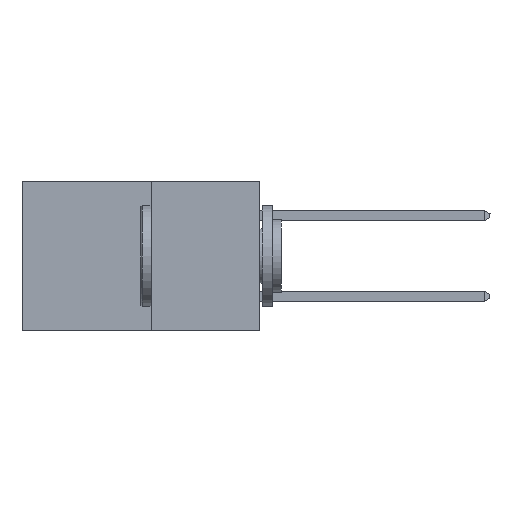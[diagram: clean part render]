
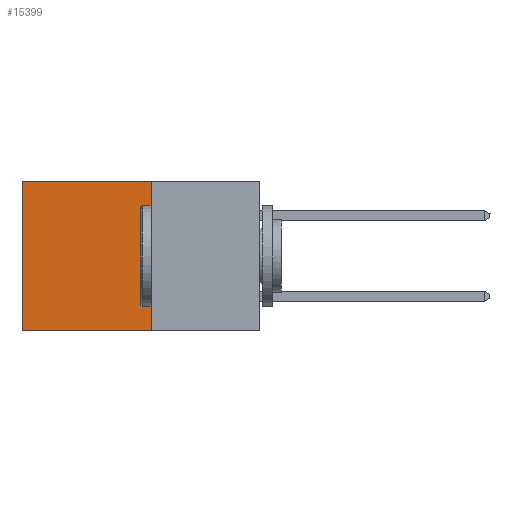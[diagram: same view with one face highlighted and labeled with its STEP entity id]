
A CAD part, left-side view. The second image highlights one B-rep face of the part: STEP entity #15399.
In plain terms, the highlighted planar face has unit normal (-1, 0, 0).
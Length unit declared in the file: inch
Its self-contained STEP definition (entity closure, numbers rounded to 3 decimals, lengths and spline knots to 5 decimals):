
#458 = DIRECTION ( 'NONE',  ( 0., 0., -1. ) ) ;
#594 = VERTEX_POINT ( 'NONE', #15744 ) ;
#2155 = DIRECTION ( 'NONE',  ( 0., 1., 0. ) ) ;
#2899 = LINE ( 'NONE', #18037, #20025 ) ;
#4515 = VERTEX_POINT ( 'NONE', #9494 ) ;
#5535 = LINE ( 'NONE', #11780, #16929 ) ;
#6347 = VECTOR ( 'NONE', #9469, 39.37008 ) ;
#6764 = DIRECTION ( 'NONE',  ( 0., 0., -1. ) ) ;
#6783 = ORIENTED_EDGE ( 'NONE', *, *, #17191, .T. ) ;
#6915 = LINE ( 'NONE', #15033, #10724 ) ;
#6976 = PLANE ( 'NONE',  #14685 ) ;
#7483 = EDGE_CURVE ( 'NONE', #8449, #4515, #5535, .T. ) ;
#7551 = ORIENTED_EDGE ( 'NONE', *, *, #7483, .F. ) ;
#7820 = CARTESIAN_POINT ( 'NONE',  ( 0.277, 0.27, -0.37 ) ) ;
#8366 = CARTESIAN_POINT ( 'NONE',  ( 0.277, 0.27, -0.37 ) ) ;
#8449 = VERTEX_POINT ( 'NONE', #8366 ) ;
#8558 = ORIENTED_EDGE ( 'NONE', *, *, #10675, .T. ) ;
#8625 = CARTESIAN_POINT ( 'NONE',  ( 0.277, 0.27, -0.37 ) ) ;
#9253 = VERTEX_POINT ( 'NONE', #14214 ) ;
#9469 = DIRECTION ( 'NONE',  ( 0., 0., -1. ) ) ;
#9494 = CARTESIAN_POINT ( 'NONE',  ( 0.277, 0.59, -0.37 ) ) ;
#10244 = DIRECTION ( 'NONE',  ( 1., 0., 0. ) ) ;
#10675 = EDGE_CURVE ( 'NONE', #594, #9253, #6915, .T. ) ;
#10724 = VECTOR ( 'NONE', #2155, 39.37008 ) ;
#11780 = CARTESIAN_POINT ( 'NONE',  ( 0.277, 0.27, -0.37 ) ) ;
#12217 = DIRECTION ( 'NONE',  ( 0., 1., 0. ) ) ;
#13664 = EDGE_CURVE ( 'NONE', #594, #8449, #19206, .T. ) ;
#14214 = CARTESIAN_POINT ( 'NONE',  ( 0.277, 0.59, 0. ) ) ;
#14685 = AXIS2_PLACEMENT_3D ( 'NONE', #8625, #10244, #458 ) ;
#15033 = CARTESIAN_POINT ( 'NONE',  ( 0.277, 0.27, 0. ) ) ;
#15399 = ADVANCED_FACE ( 'NONE', ( #20100 ), #6976, .F. ) ;
#15744 = CARTESIAN_POINT ( 'NONE',  ( 0.277, 0.27, 0. ) ) ;
#16929 = VECTOR ( 'NONE', #12217, 39.37008 ) ;
#17048 = EDGE_LOOP ( 'NONE', ( #6783, #7551, #18990, #8558 ) ) ;
#17191 = EDGE_CURVE ( 'NONE', #9253, #4515, #2899, .T. ) ;
#18037 = CARTESIAN_POINT ( 'NONE',  ( 0.277, 0.59, -0.37 ) ) ;
#18990 = ORIENTED_EDGE ( 'NONE', *, *, #13664, .F. ) ;
#19206 = LINE ( 'NONE', #7820, #6347 ) ;
#20025 = VECTOR ( 'NONE', #6764, 39.37008 ) ;
#20100 = FACE_OUTER_BOUND ( 'NONE', #17048, .T. ) ;
